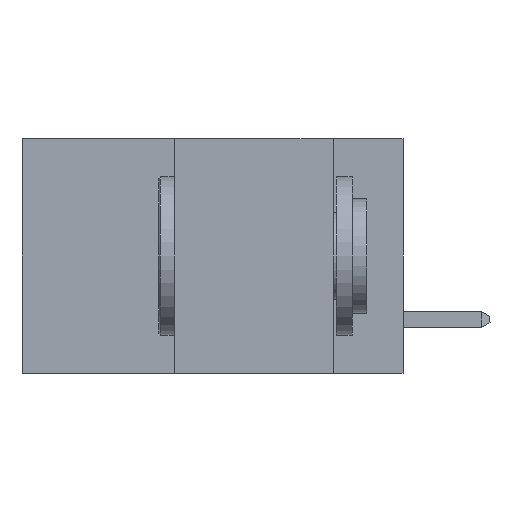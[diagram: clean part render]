
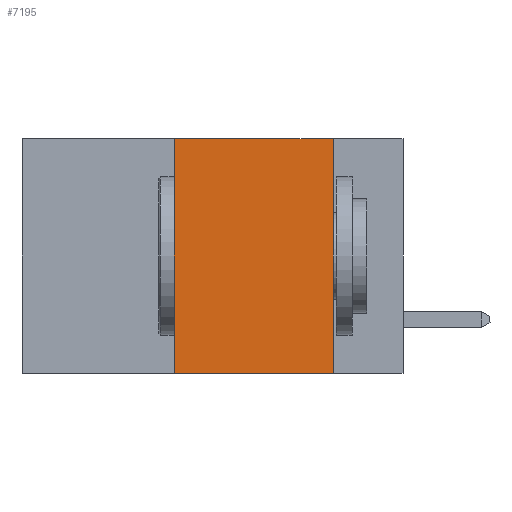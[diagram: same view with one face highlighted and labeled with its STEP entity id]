
A CAD part, left-side view. The second image highlights one B-rep face of the part: STEP entity #7195.
In plain terms, the highlighted planar face has unit normal (-1, 0, 0).
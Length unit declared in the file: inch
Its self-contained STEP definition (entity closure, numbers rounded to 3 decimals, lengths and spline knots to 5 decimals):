
#1105 = DIRECTION ( 'NONE',  ( 1., 0., 0. ) ) ;
#2177 = CARTESIAN_POINT ( 'NONE',  ( 0., 0.11, 0. ) ) ;
#3952 = VECTOR ( 'NONE', #27325, 39.37008 ) ;
#4488 = AXIS2_PLACEMENT_3D ( 'NONE', #16694, #1105, #19306 ) ;
#5814 = ORIENTED_EDGE ( 'NONE', *, *, #9696, .F. ) ;
#7195 = ADVANCED_FACE ( 'NONE', ( #7332 ), #32219, .F. ) ;
#7235 = VECTOR ( 'NONE', #18748, 39.37008 ) ;
#7332 = FACE_OUTER_BOUND ( 'NONE', #9750, .T. ) ;
#7883 = ORIENTED_EDGE ( 'NONE', *, *, #8115, .F. ) ;
#8115 = EDGE_CURVE ( 'NONE', #8458, #12891, #11752, .T. ) ;
#8352 = CARTESIAN_POINT ( 'NONE',  ( 0., 0.6, 0. ) ) ;
#8458 = VERTEX_POINT ( 'NONE', #30940 ) ;
#9696 = EDGE_CURVE ( 'NONE', #19087, #30695, #23268, .T. ) ;
#9750 = EDGE_LOOP ( 'NONE', ( #7883, #15738, #5814, #21721 ) ) ;
#11186 = EDGE_CURVE ( 'NONE', #30695, #8458, #14167, .T. ) ;
#11700 = EDGE_CURVE ( 'NONE', #19087, #12891, #31620, .T. ) ;
#11752 = LINE ( 'NONE', #2177, #17905 ) ;
#12891 = VERTEX_POINT ( 'NONE', #29299 ) ;
#12921 = CARTESIAN_POINT ( 'NONE',  ( 0., 0.36, 0. ) ) ;
#14167 = LINE ( 'NONE', #8352, #7235 ) ;
#15738 = ORIENTED_EDGE ( 'NONE', *, *, #11186, .F. ) ;
#16694 = CARTESIAN_POINT ( 'NONE',  ( 0., 0.6, 0. ) ) ;
#17790 = DIRECTION ( 'NONE',  ( 0., 0., -1. ) ) ;
#17905 = VECTOR ( 'NONE', #17790, 39.37008 ) ;
#18748 = DIRECTION ( 'NONE',  ( 0., -1., 0. ) ) ;
#19087 = VERTEX_POINT ( 'NONE', #33032 ) ;
#19306 = DIRECTION ( 'NONE',  ( 0., 0., -1. ) ) ;
#21721 = ORIENTED_EDGE ( 'NONE', *, *, #11700, .T. ) ;
#22457 = VECTOR ( 'NONE', #28505, 39.37008 ) ;
#23268 = LINE ( 'NONE', #12921, #22457 ) ;
#27325 = DIRECTION ( 'NONE',  ( 0., -1., 0. ) ) ;
#28505 = DIRECTION ( 'NONE',  ( 0., 0., 1. ) ) ;
#29299 = CARTESIAN_POINT ( 'NONE',  ( 0., 0.11, -0.37 ) ) ;
#30695 = VERTEX_POINT ( 'NONE', #32259 ) ;
#30940 = CARTESIAN_POINT ( 'NONE',  ( 0., 0.11, 0. ) ) ;
#31620 = LINE ( 'NONE', #32310, #3952 ) ;
#32219 = PLANE ( 'NONE',  #4488 ) ;
#32259 = CARTESIAN_POINT ( 'NONE',  ( 0., 0.36, 0. ) ) ;
#32310 = CARTESIAN_POINT ( 'NONE',  ( 0., 0.6, -0.37 ) ) ;
#33032 = CARTESIAN_POINT ( 'NONE',  ( 0., 0.36, -0.37 ) ) ;
